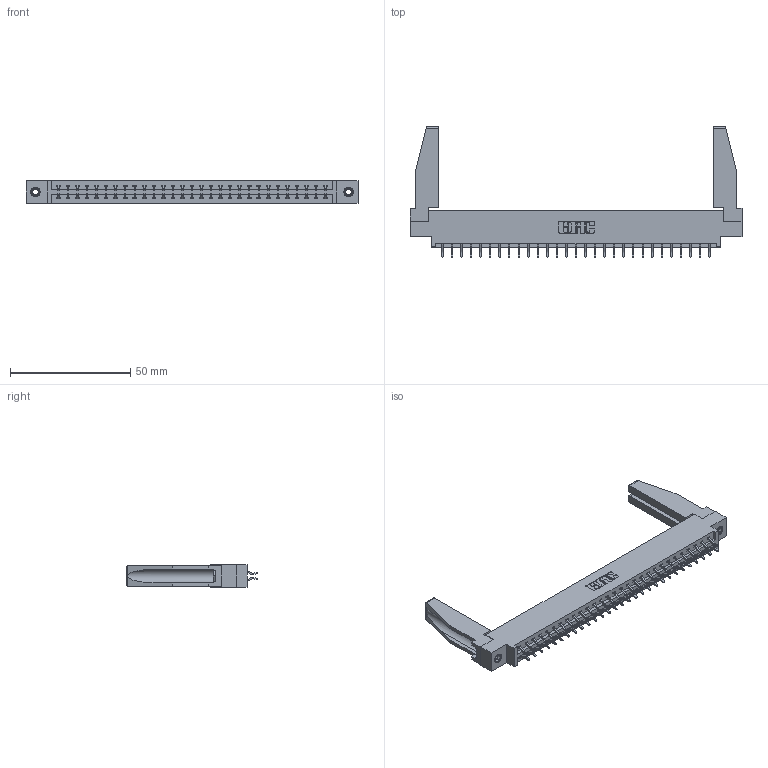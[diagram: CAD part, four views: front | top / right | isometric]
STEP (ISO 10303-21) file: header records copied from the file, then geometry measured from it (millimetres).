
FILE_DESCRIPTION (( 'STEP AP203' ), '1' );
FILE_NAME ('387-058-556-878.STEP', '2019-10-19T10:04:33', ( '' ), ( '' ), 'SwSTEP 2.0', 'SolidWorks 2016', '' );
FILE_SCHEMA (( 'CONFIG_CONTROL_DESIGN' ));
Length unit declared in the file: inch
Products named in the file (5): 345-250-001_345-250-001-102; 337 Part_0.170 Offset - 0.156 Dia-TI; 307-220-078; 345-292-001_556 Tail; 387-058-556-878
Assembly tree (63 placements, depth 2):
  387-058-556-878
    337 Part_0.170 Offset - 0.156 Dia-TI
    345-292-001_556 Tail  x58
    345-250-001_345-250-001-102  x2
    307-220-078  x2
Bounding box: 137.92 x 54.37 x 9.4 mm (x, y, z)
Volume: 18235.8 mm3; surface area: 19852 mm2
Topology: 63 solids, 63 shells, 3728 faces, 11035 edges, 7270 vertices
Faces by surface type: plane 2594, cylinder 1118, cone 12, torus 4
Entity records: 26958 total; most frequent: CARTESIAN_POINT 4568, ORIENTED_EDGE 4448, DIRECTION 3904, EDGE_CURVE 2224, LINE 2050, VECTOR 2050, VERTEX_POINT 1476, AXIS2_PLACEMENT_3D 927
